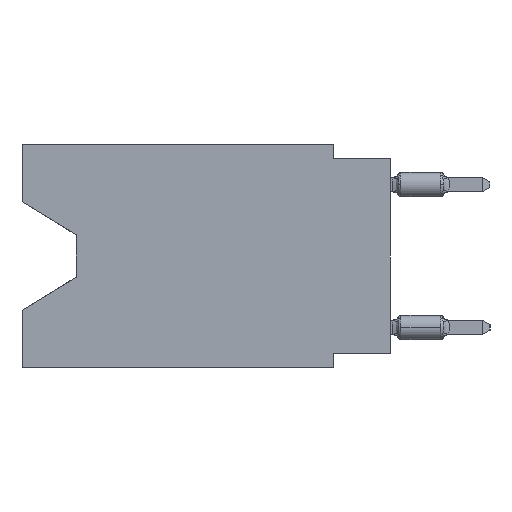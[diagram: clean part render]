
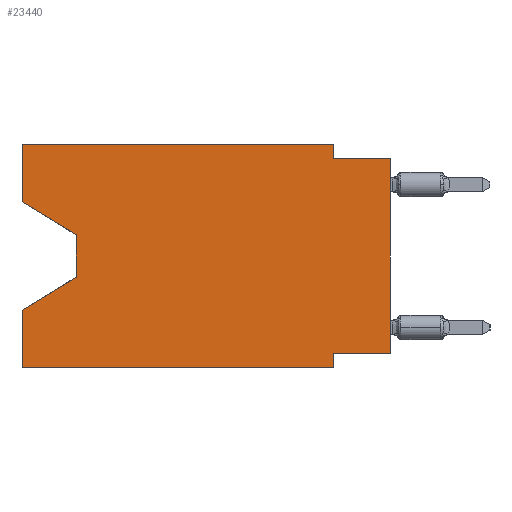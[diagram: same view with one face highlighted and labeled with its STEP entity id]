
A CAD part, left-side view. The second image highlights one B-rep face of the part: STEP entity #23440.
In plain terms, the highlighted planar face has unit normal (-1, 0, 0).
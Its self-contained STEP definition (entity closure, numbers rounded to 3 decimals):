
#1203 = CARTESIAN_POINT ( 'NONE',  ( 0., 13.97, -5.893 ) ) ;
#1417 = EDGE_LOOP ( 'NONE', ( #14625, #32188, #43158, #3737, #28964, #22605, #8500, #21546, #38784, #36331, #28944, #9916 ) ) ;
#1699 = CARTESIAN_POINT ( 'NONE',  ( 0., 16.383, -2.546 ) ) ;
#2441 = CARTESIAN_POINT ( 'NONE',  ( 0., 16.383, 0. ) ) ;
#2665 = VECTOR ( 'NONE', #32168, 1000. ) ;
#2746 = EDGE_CURVE ( 'NONE', #14242, #14169, #12673, .T. ) ;
#3737 = ORIENTED_EDGE ( 'NONE', *, *, #17666, .F. ) ;
#4246 = FACE_OUTER_BOUND ( 'NONE', #1417, .T. ) ;
#4942 = EDGE_CURVE ( 'NONE', #15386, #23028, #15292, .T. ) ;
#5286 = EDGE_CURVE ( 'NONE', #34247, #38543, #17753, .T. ) ;
#5297 = VECTOR ( 'NONE', #33003, 1000. ) ;
#6494 = LINE ( 'NONE', #18023, #30546 ) ;
#7152 = VERTEX_POINT ( 'NONE', #21401 ) ;
#7278 = DIRECTION ( 'NONE',  ( 0., -1., 0. ) ) ;
#7761 = DIRECTION ( 'NONE',  ( 0., 0., -1. ) ) ;
#8029 = VECTOR ( 'NONE', #7278, 1000. ) ;
#8500 = ORIENTED_EDGE ( 'NONE', *, *, #5286, .F. ) ;
#8711 = LINE ( 'NONE', #1203, #28083 ) ;
#9214 = DIRECTION ( 'NONE',  ( 0., 0.855, -0.519 ) ) ;
#9429 = EDGE_CURVE ( 'NONE', #14169, #39215, #34551, .T. ) ;
#9848 = CARTESIAN_POINT ( 'NONE',  ( 0., 0., -0.635 ) ) ;
#9916 = ORIENTED_EDGE ( 'NONE', *, *, #10102, .F. ) ;
#10102 = EDGE_CURVE ( 'NONE', #40870, #42642, #36714, .T. ) ;
#10269 = DIRECTION ( 'NONE',  ( 0., 0., 1. ) ) ;
#10578 = VECTOR ( 'NONE', #18340, 1000. ) ;
#10841 = CARTESIAN_POINT ( 'NONE',  ( 0., 2.54, -9.906 ) ) ;
#11054 = CARTESIAN_POINT ( 'NONE',  ( 0., 16.383, -9.906 ) ) ;
#11315 = DIRECTION ( 'NONE',  ( 0., 0., -1. ) ) ;
#11778 = PLANE ( 'NONE',  #48275 ) ;
#12219 = VECTOR ( 'NONE', #12954, 1000. ) ;
#12673 = LINE ( 'NONE', #31192, #2665 ) ;
#12744 = VERTEX_POINT ( 'NONE', #42963 ) ;
#12880 = LINE ( 'NONE', #28140, #47792 ) ;
#12954 = DIRECTION ( 'NONE',  ( 0., -0.855, -0.519 ) ) ;
#13894 = CARTESIAN_POINT ( 'NONE',  ( 0., 0., 0. ) ) ;
#14169 = VERTEX_POINT ( 'NONE', #28954 ) ;
#14242 = VERTEX_POINT ( 'NONE', #45427 ) ;
#14625 = ORIENTED_EDGE ( 'NONE', *, *, #36000, .T. ) ;
#15080 = CARTESIAN_POINT ( 'NONE',  ( 0., 13.97, -4.013 ) ) ;
#15292 = LINE ( 'NONE', #11054, #8029 ) ;
#15386 = VERTEX_POINT ( 'NONE', #46769 ) ;
#17666 = EDGE_CURVE ( 'NONE', #15386, #28631, #6494, .T. ) ;
#17753 = LINE ( 'NONE', #32520, #5297 ) ;
#18023 = CARTESIAN_POINT ( 'NONE',  ( 0., 16.383, 0. ) ) ;
#18340 = DIRECTION ( 'NONE',  ( 0., 0., -1. ) ) ;
#19012 = CARTESIAN_POINT ( 'NONE',  ( 0., 0., -9.271 ) ) ;
#19072 = CARTESIAN_POINT ( 'NONE',  ( 0., 0., -0.635 ) ) ;
#19453 = VECTOR ( 'NONE', #11315, 1000. ) ;
#19527 = CARTESIAN_POINT ( 'NONE',  ( 0., 16.383, 0. ) ) ;
#20464 = LINE ( 'NONE', #28955, #12219 ) ;
#21401 = CARTESIAN_POINT ( 'NONE',  ( 0., 13.97, -4.013 ) ) ;
#21546 = ORIENTED_EDGE ( 'NONE', *, *, #34899, .T. ) ;
#22605 = ORIENTED_EDGE ( 'NONE', *, *, #43134, .F. ) ;
#23028 = VERTEX_POINT ( 'NONE', #29674 ) ;
#23440 = ADVANCED_FACE ( 'NONE', ( #4246 ), #11778, .F. ) ;
#25400 = DIRECTION ( 'NONE',  ( 0., 0., 1. ) ) ;
#25715 = DIRECTION ( 'NONE',  ( 0., 0., 1. ) ) ;
#28083 = VECTOR ( 'NONE', #9214, 1000. ) ;
#28140 = CARTESIAN_POINT ( 'NONE',  ( 0., 16.383, 0. ) ) ;
#28631 = VERTEX_POINT ( 'NONE', #29480 ) ;
#28944 = ORIENTED_EDGE ( 'NONE', *, *, #31888, .F. ) ;
#28954 = CARTESIAN_POINT ( 'NONE',  ( 0., 2.54, -0.635 ) ) ;
#28955 = CARTESIAN_POINT ( 'NONE',  ( 0., 16.383, -2.546 ) ) ;
#28964 = ORIENTED_EDGE ( 'NONE', *, *, #4942, .T. ) ;
#29480 = CARTESIAN_POINT ( 'NONE',  ( 0., 16.383, -7.36 ) ) ;
#29602 = LINE ( 'NONE', #10841, #10578 ) ;
#29674 = CARTESIAN_POINT ( 'NONE',  ( 0., 2.54, -9.906 ) ) ;
#30546 = VECTOR ( 'NONE', #10269, 1000. ) ;
#31034 = DIRECTION ( 'NONE',  ( 1., 0., 0. ) ) ;
#31192 = CARTESIAN_POINT ( 'NONE',  ( 0., 2.54, 0. ) ) ;
#31888 = EDGE_CURVE ( 'NONE', #42642, #14242, #12880, .T. ) ;
#32168 = DIRECTION ( 'NONE',  ( 0., 0., -1. ) ) ;
#32188 = ORIENTED_EDGE ( 'NONE', *, *, #42045, .T. ) ;
#32520 = CARTESIAN_POINT ( 'NONE',  ( 0., 0., -9.271 ) ) ;
#32627 = DIRECTION ( 'NONE',  ( 0., -1., 0. ) ) ;
#32884 = LINE ( 'NONE', #13894, #45659 ) ;
#33003 = DIRECTION ( 'NONE',  ( 0., 1., 0. ) ) ;
#33334 = LINE ( 'NONE', #15080, #19453 ) ;
#34247 = VERTEX_POINT ( 'NONE', #19012 ) ;
#34289 = VECTOR ( 'NONE', #42059, 1000. ) ;
#34551 = LINE ( 'NONE', #19072, #34289 ) ;
#34899 = EDGE_CURVE ( 'NONE', #34247, #39215, #32884, .T. ) ;
#36000 = EDGE_CURVE ( 'NONE', #40870, #7152, #20464, .T. ) ;
#36331 = ORIENTED_EDGE ( 'NONE', *, *, #2746, .F. ) ;
#36714 = LINE ( 'NONE', #2441, #45872 ) ;
#38543 = VERTEX_POINT ( 'NONE', #41280 ) ;
#38784 = ORIENTED_EDGE ( 'NONE', *, *, #9429, .F. ) ;
#39215 = VERTEX_POINT ( 'NONE', #9848 ) ;
#39701 = EDGE_CURVE ( 'NONE', #12744, #28631, #8711, .T. ) ;
#40418 = CARTESIAN_POINT ( 'NONE',  ( 0., 16.383, 0. ) ) ;
#40870 = VERTEX_POINT ( 'NONE', #1699 ) ;
#41280 = CARTESIAN_POINT ( 'NONE',  ( 0., 2.54, -9.271 ) ) ;
#42045 = EDGE_CURVE ( 'NONE', #7152, #12744, #33334, .T. ) ;
#42059 = DIRECTION ( 'NONE',  ( 0., -1., 0. ) ) ;
#42642 = VERTEX_POINT ( 'NONE', #40418 ) ;
#42963 = CARTESIAN_POINT ( 'NONE',  ( 0., 13.97, -5.893 ) ) ;
#43134 = EDGE_CURVE ( 'NONE', #38543, #23028, #29602, .T. ) ;
#43158 = ORIENTED_EDGE ( 'NONE', *, *, #39701, .T. ) ;
#45427 = CARTESIAN_POINT ( 'NONE',  ( 0., 2.54, 0. ) ) ;
#45659 = VECTOR ( 'NONE', #25400, 1000. ) ;
#45872 = VECTOR ( 'NONE', #25715, 1000. ) ;
#46769 = CARTESIAN_POINT ( 'NONE',  ( 0., 16.383, -9.906 ) ) ;
#47792 = VECTOR ( 'NONE', #32627, 1000. ) ;
#48275 = AXIS2_PLACEMENT_3D ( 'NONE', #19527, #31034, #7761 ) ;
